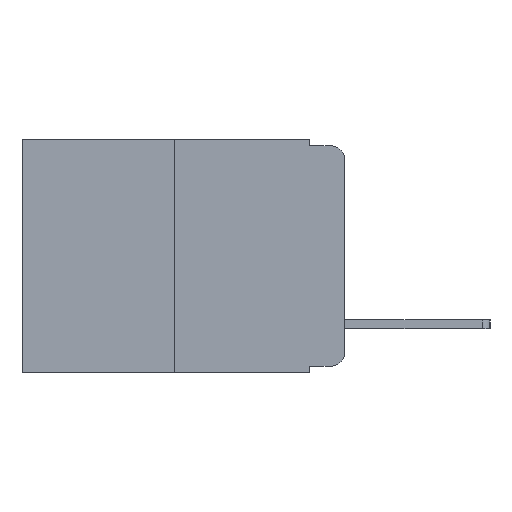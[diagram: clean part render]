
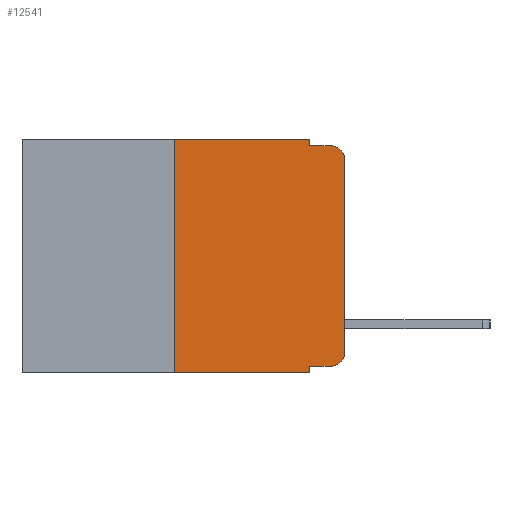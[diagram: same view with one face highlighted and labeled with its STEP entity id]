
A CAD part, left-side view. The second image highlights one B-rep face of the part: STEP entity #12541.
In plain terms, the highlighted planar face has unit normal (-1, 0, 0).
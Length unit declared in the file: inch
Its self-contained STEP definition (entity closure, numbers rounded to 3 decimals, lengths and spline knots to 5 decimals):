
#307 = VERTEX_POINT ( 'NONE', #9150 ) ;
#394 = VERTEX_POINT ( 'NONE', #15734 ) ;
#721 = EDGE_LOOP ( 'NONE', ( #8049, #16602, #4366, #13391, #2321, #17993, #12790, #769, #10423, #21050 ) ) ;
#769 = ORIENTED_EDGE ( 'NONE', *, *, #2118, .F. ) ;
#1302 = DIRECTION ( 'NONE',  ( -1., 0., 0. ) ) ;
#1492 = VECTOR ( 'NONE', #12505, 39.37008 ) ;
#1787 = LINE ( 'NONE', #20775, #6228 ) ;
#1836 = LINE ( 'NONE', #14542, #5697 ) ;
#2118 = EDGE_CURVE ( 'NONE', #307, #4906, #1836, .T. ) ;
#2199 = LINE ( 'NONE', #5065, #10964 ) ;
#2321 = ORIENTED_EDGE ( 'NONE', *, *, #22970, .F. ) ;
#2375 = CARTESIAN_POINT ( 'NONE',  ( 0., 0.473, 0. ) ) ;
#2512 = VECTOR ( 'NONE', #4292, 39.37008 ) ;
#2723 = AXIS2_PLACEMENT_3D ( 'NONE', #7831, #20822, #9784 ) ;
#2974 = EDGE_CURVE ( 'NONE', #5027, #4823, #1787, .T. ) ;
#3314 = AXIS2_PLACEMENT_3D ( 'NONE', #12491, #1302, #14374 ) ;
#3738 = DIRECTION ( 'NONE',  ( -1., 0., 0. ) ) ;
#3754 = CARTESIAN_POINT ( 'NONE',  ( 0., 0.02, -0.313 ) ) ;
#4176 = AXIS2_PLACEMENT_3D ( 'NONE', #3754, #3738, #8719 ) ;
#4197 = PLANE ( 'NONE',  #2723 ) ;
#4240 = EDGE_CURVE ( 'NONE', #21575, #20933, #23086, .T. ) ;
#4258 = VERTEX_POINT ( 'NONE', #5729 ) ;
#4292 = DIRECTION ( 'NONE',  ( 0., -1., 0. ) ) ;
#4352 = VERTEX_POINT ( 'NONE', #5866 ) ;
#4366 = ORIENTED_EDGE ( 'NONE', *, *, #2974, .F. ) ;
#4823 = VERTEX_POINT ( 'NONE', #8112 ) ;
#4906 = VERTEX_POINT ( 'NONE', #9231 ) ;
#5024 = CARTESIAN_POINT ( 'NONE',  ( 0., 0.25, 0. ) ) ;
#5027 = VERTEX_POINT ( 'NONE', #23742 ) ;
#5065 = CARTESIAN_POINT ( 'NONE',  ( 0., 0.473, -0.343 ) ) ;
#5697 = VECTOR ( 'NONE', #23785, 39.37008 ) ;
#5729 = CARTESIAN_POINT ( 'NONE',  ( 0., 0.25, -0.343 ) ) ;
#5866 = CARTESIAN_POINT ( 'NONE',  ( 0., 0.051, 0. ) ) ;
#6083 = VERTEX_POINT ( 'NONE', #5024 ) ;
#6228 = VECTOR ( 'NONE', #20789, 39.37008 ) ;
#6502 = LINE ( 'NONE', #21640, #1492 ) ;
#6993 = DIRECTION ( 'NONE',  ( 0., 0., 1. ) ) ;
#7777 = FACE_OUTER_BOUND ( 'NONE', #721, .T. ) ;
#7831 = CARTESIAN_POINT ( 'NONE',  ( 0., 0.473, 0. ) ) ;
#8049 = ORIENTED_EDGE ( 'NONE', *, *, #12914, .T. ) ;
#8112 = CARTESIAN_POINT ( 'NONE',  ( 0., 0.02, -0.01 ) ) ;
#8719 = DIRECTION ( 'NONE',  ( 0., 0., -1. ) ) ;
#9150 = CARTESIAN_POINT ( 'NONE',  ( 0., 0.051, -0.333 ) ) ;
#9231 = CARTESIAN_POINT ( 'NONE',  ( 0., 0.051, -0.343 ) ) ;
#9784 = DIRECTION ( 'NONE',  ( 0., 0., -1. ) ) ;
#10263 = LINE ( 'NONE', #11181, #19469 ) ;
#10423 = ORIENTED_EDGE ( 'NONE', *, *, #18886, .T. ) ;
#10964 = VECTOR ( 'NONE', #21639, 39.37008 ) ;
#11181 = CARTESIAN_POINT ( 'NONE',  ( 0., 0.051, 0. ) ) ;
#12491 = CARTESIAN_POINT ( 'NONE',  ( 0., 0.02, -0.03 ) ) ;
#12505 = DIRECTION ( 'NONE',  ( 0., 0., 1. ) ) ;
#12541 = ADVANCED_FACE ( 'NONE', ( #7777 ), #4197, .F. ) ;
#12790 = ORIENTED_EDGE ( 'NONE', *, *, #22624, .T. ) ;
#12914 = EDGE_CURVE ( 'NONE', #20933, #394, #19903, .T. ) ;
#13069 = DIRECTION ( 'NONE',  ( 0., 0., -1. ) ) ;
#13391 = ORIENTED_EDGE ( 'NONE', *, *, #19414, .F. ) ;
#14374 = DIRECTION ( 'NONE',  ( 0., 0., -1. ) ) ;
#14414 = CARTESIAN_POINT ( 'NONE',  ( 0., 0., 0. ) ) ;
#14542 = CARTESIAN_POINT ( 'NONE',  ( 0., 0.051, 0. ) ) ;
#14849 = EDGE_CURVE ( 'NONE', #4258, #6083, #6502, .T. ) ;
#15046 = VECTOR ( 'NONE', #6993, 39.37008 ) ;
#15734 = CARTESIAN_POINT ( 'NONE',  ( 0., 0., -0.03 ) ) ;
#16602 = ORIENTED_EDGE ( 'NONE', *, *, #19234, .T. ) ;
#17319 = LINE ( 'NONE', #2375, #2512 ) ;
#17498 = VECTOR ( 'NONE', #17867, 39.37008 ) ;
#17613 = CARTESIAN_POINT ( 'NONE',  ( 0., 0.02, -0.333 ) ) ;
#17867 = DIRECTION ( 'NONE',  ( 0., -1., 0. ) ) ;
#17993 = ORIENTED_EDGE ( 'NONE', *, *, #14849, .F. ) ;
#18886 = EDGE_CURVE ( 'NONE', #307, #21575, #22342, .T. ) ;
#19188 = CIRCLE ( 'NONE', #3314, 0.02 ) ;
#19234 = EDGE_CURVE ( 'NONE', #394, #4823, #19188, .T. ) ;
#19414 = EDGE_CURVE ( 'NONE', #4352, #5027, #10263, .T. ) ;
#19469 = VECTOR ( 'NONE', #13069, 39.37008 ) ;
#19624 = CARTESIAN_POINT ( 'NONE',  ( 0., 0.051, -0.333 ) ) ;
#19903 = LINE ( 'NONE', #14414, #15046 ) ;
#20775 = CARTESIAN_POINT ( 'NONE',  ( 0., 0.051, -0.01 ) ) ;
#20789 = DIRECTION ( 'NONE',  ( 0., -1., 0. ) ) ;
#20822 = DIRECTION ( 'NONE',  ( 1., 0., 0. ) ) ;
#20933 = VERTEX_POINT ( 'NONE', #22711 ) ;
#21050 = ORIENTED_EDGE ( 'NONE', *, *, #4240, .T. ) ;
#21575 = VERTEX_POINT ( 'NONE', #17613 ) ;
#21639 = DIRECTION ( 'NONE',  ( 0., -1., 0. ) ) ;
#21640 = CARTESIAN_POINT ( 'NONE',  ( 0., 0.25, 0. ) ) ;
#22342 = LINE ( 'NONE', #19624, #17498 ) ;
#22624 = EDGE_CURVE ( 'NONE', #4258, #4906, #2199, .T. ) ;
#22711 = CARTESIAN_POINT ( 'NONE',  ( 0., 0., -0.313 ) ) ;
#22970 = EDGE_CURVE ( 'NONE', #6083, #4352, #17319, .T. ) ;
#23086 = CIRCLE ( 'NONE', #4176, 0.02 ) ;
#23742 = CARTESIAN_POINT ( 'NONE',  ( 0., 0.051, -0.01 ) ) ;
#23785 = DIRECTION ( 'NONE',  ( 0., 0., -1. ) ) ;
